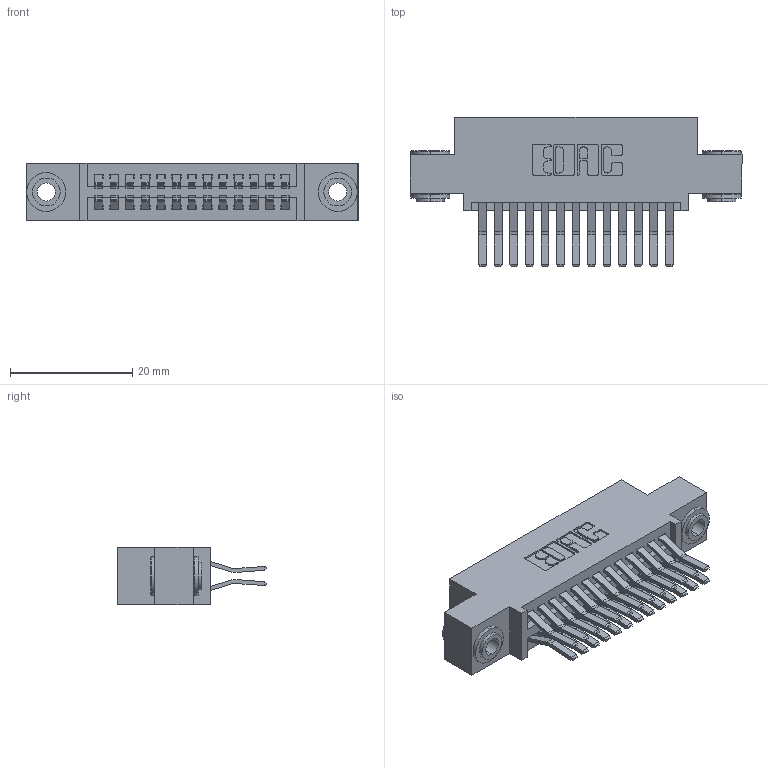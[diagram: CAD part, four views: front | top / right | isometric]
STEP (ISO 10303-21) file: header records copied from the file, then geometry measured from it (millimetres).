
FILE_DESCRIPTION (( 'STEP AP203' ), '1' );
FILE_NAME ('395-026-560-503.STEP', '2018-11-10T03:39:34', ( '' ), ( '' ), 'SwSTEP 2.0', 'SolidWorks 2016', '' );
FILE_SCHEMA (( 'CONFIG_CONTROL_DESIGN' ));
Length unit declared in the file: inch
Products named in the file (4): 395-026-560-503; 345-292-001_560 Tail; 345 Part_0.110 Offset - 0.156 Dia-TH; 345-250-002_345-250-002-102
Assembly tree (29 placements, depth 2):
  395-026-560-503
    345 Part_0.110 Offset - 0.156 Dia-TH
    345-292-001_560 Tail  x26
    345-250-002_345-250-002-102  x2
Bounding box: 54.23 x 24.45 x 9.4 mm (x, y, z)
Volume: 5115.1 mm3; surface area: 7735.4 mm2
Topology: 29 solids, 29 shells, 1520 faces, 4459 edges, 2934 vertices
Faces by surface type: plane 952, cylinder 560, cone 8
Entity records: 14974 total; most frequent: CARTESIAN_POINT 2515, ORIENTED_EDGE 2442, DIRECTION 2287, EDGE_CURVE 1221, LINE 1009, VECTOR 1009, VERTEX_POINT 810, AXIS2_PLACEMENT_3D 639
